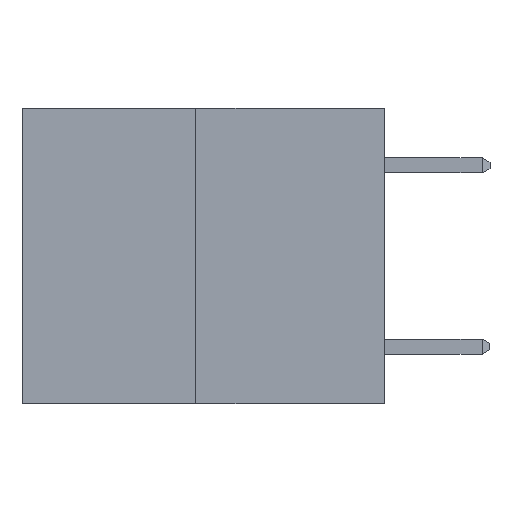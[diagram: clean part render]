
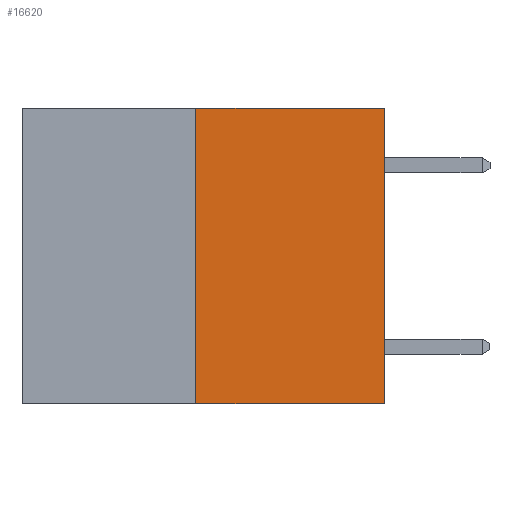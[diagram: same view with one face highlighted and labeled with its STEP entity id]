
A CAD part, left-side view. The second image highlights one B-rep face of the part: STEP entity #16620.
In plain terms, the highlighted planar face has unit normal (-1, 0, 0).
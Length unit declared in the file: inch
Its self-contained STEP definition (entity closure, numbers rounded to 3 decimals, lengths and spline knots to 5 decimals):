
#82 = ORIENTED_EDGE ( 'NONE', *, *, #15900, .F. ) ;
#394 = PLANE ( 'NONE',  #1518 ) ;
#624 = CARTESIAN_POINT ( 'NONE',  ( 0., 0.6, 0. ) ) ;
#1518 = AXIS2_PLACEMENT_3D ( 'NONE', #624, #1782, #11057 ) ;
#1782 = DIRECTION ( 'NONE',  ( 1., 0., 0. ) ) ;
#1968 = EDGE_LOOP ( 'NONE', ( #15731, #15186, #4108, #82 ) ) ;
#2005 = EDGE_CURVE ( 'NONE', #5358, #13709, #15645, .T. ) ;
#2757 = LINE ( 'NONE', #5600, #2966 ) ;
#2966 = VECTOR ( 'NONE', #6781, 39.37008 ) ;
#3443 = VECTOR ( 'NONE', #15374, 39.37008 ) ;
#3728 = CARTESIAN_POINT ( 'NONE',  ( 0., 0.312, 0. ) ) ;
#4108 = ORIENTED_EDGE ( 'NONE', *, *, #16554, .T. ) ;
#4427 = VECTOR ( 'NONE', #6542, 39.37008 ) ;
#5358 = VERTEX_POINT ( 'NONE', #10714 ) ;
#5600 = CARTESIAN_POINT ( 'NONE',  ( 0., 0., 0. ) ) ;
#5929 = EDGE_CURVE ( 'NONE', #5358, #8496, #8586, .T. ) ;
#6269 = CARTESIAN_POINT ( 'NONE',  ( 0., 0.312, -0.49 ) ) ;
#6542 = DIRECTION ( 'NONE',  ( 0., -1., 0. ) ) ;
#6650 = CARTESIAN_POINT ( 'NONE',  ( 0., 0.6, -0.49 ) ) ;
#6781 = DIRECTION ( 'NONE',  ( 0., 0., 1. ) ) ;
#7395 = CARTESIAN_POINT ( 'NONE',  ( 0., 0., -0.49 ) ) ;
#8131 = VERTEX_POINT ( 'NONE', #16826 ) ;
#8183 = DIRECTION ( 'NONE',  ( 0., -1., 0. ) ) ;
#8496 = VERTEX_POINT ( 'NONE', #3728 ) ;
#8586 = LINE ( 'NONE', #6269, #3443 ) ;
#9908 = FACE_OUTER_BOUND ( 'NONE', #1968, .T. ) ;
#10714 = CARTESIAN_POINT ( 'NONE',  ( 0., 0.312, -0.49 ) ) ;
#11057 = DIRECTION ( 'NONE',  ( 0., 0., -1. ) ) ;
#12296 = CARTESIAN_POINT ( 'NONE',  ( 0., 0.6, 0. ) ) ;
#12997 = VECTOR ( 'NONE', #8183, 39.37008 ) ;
#13709 = VERTEX_POINT ( 'NONE', #7395 ) ;
#15186 = ORIENTED_EDGE ( 'NONE', *, *, #2005, .T. ) ;
#15374 = DIRECTION ( 'NONE',  ( 0., 0., 1. ) ) ;
#15645 = LINE ( 'NONE', #6650, #4427 ) ;
#15731 = ORIENTED_EDGE ( 'NONE', *, *, #5929, .F. ) ;
#15900 = EDGE_CURVE ( 'NONE', #8496, #8131, #16448, .T. ) ;
#16448 = LINE ( 'NONE', #12296, #12997 ) ;
#16554 = EDGE_CURVE ( 'NONE', #13709, #8131, #2757, .T. ) ;
#16620 = ADVANCED_FACE ( 'NONE', ( #9908 ), #394, .F. ) ;
#16826 = CARTESIAN_POINT ( 'NONE',  ( 0., 0., 0. ) ) ;
